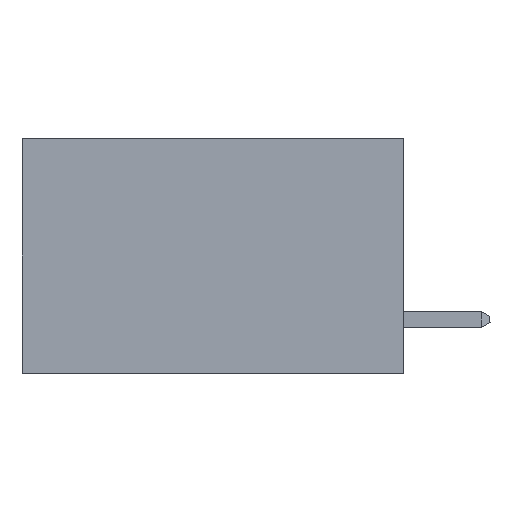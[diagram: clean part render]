
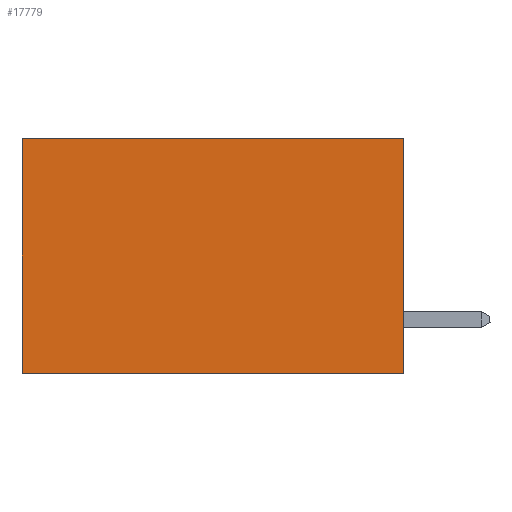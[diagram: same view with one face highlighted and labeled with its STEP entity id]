
A CAD part, left-side view. The second image highlights one B-rep face of the part: STEP entity #17779.
In plain terms, the highlighted planar face has unit normal (-1, 0, 0).
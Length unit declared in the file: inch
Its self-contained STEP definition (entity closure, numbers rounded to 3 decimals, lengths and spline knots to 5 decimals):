
#840 = DIRECTION ( 'NONE',  ( 0., 1., 0. ) ) ;
#1267 = CARTESIAN_POINT ( 'NONE',  ( 0.2875, 0., 0. ) ) ;
#1452 = LINE ( 'NONE', #3862, #44918 ) ;
#2771 = DIRECTION ( 'NONE',  ( 0., 0., -1. ) ) ;
#2837 = LINE ( 'NONE', #15222, #7184 ) ;
#3540 = VERTEX_POINT ( 'NONE', #9427 ) ;
#3862 = CARTESIAN_POINT ( 'NONE',  ( 0.2875, 0.6, 0. ) ) ;
#4524 = EDGE_CURVE ( 'NONE', #3540, #30016, #1452, .T. ) ;
#6466 = LINE ( 'NONE', #25126, #30943 ) ;
#6983 = FACE_OUTER_BOUND ( 'NONE', #30531, .T. ) ;
#7184 = VECTOR ( 'NONE', #11914, 39.37008 ) ;
#9427 = CARTESIAN_POINT ( 'NONE',  ( 0.2875, 0.6, 0. ) ) ;
#9559 = CARTESIAN_POINT ( 'NONE',  ( 0.2875, 0., 0. ) ) ;
#11879 = VERTEX_POINT ( 'NONE', #1267 ) ;
#11914 = DIRECTION ( 'NONE',  ( 0., 1., 0. ) ) ;
#15222 = CARTESIAN_POINT ( 'NONE',  ( 0.2875, 0., 0. ) ) ;
#15803 = ORIENTED_EDGE ( 'NONE', *, *, #4524, .T. ) ;
#16396 = CARTESIAN_POINT ( 'NONE',  ( 0.2875, 0.6, -0.37 ) ) ;
#17779 = ADVANCED_FACE ( 'NONE', ( #6983 ), #26897, .F. ) ;
#18603 = ORIENTED_EDGE ( 'NONE', *, *, #28014, .T. ) ;
#20095 = DIRECTION ( 'NONE',  ( 1., 0., 0. ) ) ;
#22785 = DIRECTION ( 'NONE',  ( 0., 0., -1. ) ) ;
#25126 = CARTESIAN_POINT ( 'NONE',  ( 0.2875, 0., -0.37 ) ) ;
#26897 = PLANE ( 'NONE',  #43060 ) ;
#28014 = EDGE_CURVE ( 'NONE', #11879, #3540, #2837, .T. ) ;
#28179 = DIRECTION ( 'NONE',  ( 0., 0., -1. ) ) ;
#28255 = ORIENTED_EDGE ( 'NONE', *, *, #44769, .F. ) ;
#29788 = EDGE_CURVE ( 'NONE', #32901, #30016, #6466, .T. ) ;
#30016 = VERTEX_POINT ( 'NONE', #16396 ) ;
#30531 = EDGE_LOOP ( 'NONE', ( #15803, #44039, #28255, #18603 ) ) ;
#30943 = VECTOR ( 'NONE', #840, 39.37008 ) ;
#31354 = CARTESIAN_POINT ( 'NONE',  ( 0.2875, 0., -0.37 ) ) ;
#32901 = VERTEX_POINT ( 'NONE', #31354 ) ;
#33462 = VECTOR ( 'NONE', #22785, 39.37008 ) ;
#36164 = LINE ( 'NONE', #9559, #33462 ) ;
#40854 = CARTESIAN_POINT ( 'NONE',  ( 0.2875, 0., 0. ) ) ;
#43060 = AXIS2_PLACEMENT_3D ( 'NONE', #40854, #20095, #2771 ) ;
#44039 = ORIENTED_EDGE ( 'NONE', *, *, #29788, .F. ) ;
#44769 = EDGE_CURVE ( 'NONE', #11879, #32901, #36164, .T. ) ;
#44918 = VECTOR ( 'NONE', #28179, 39.37008 ) ;
